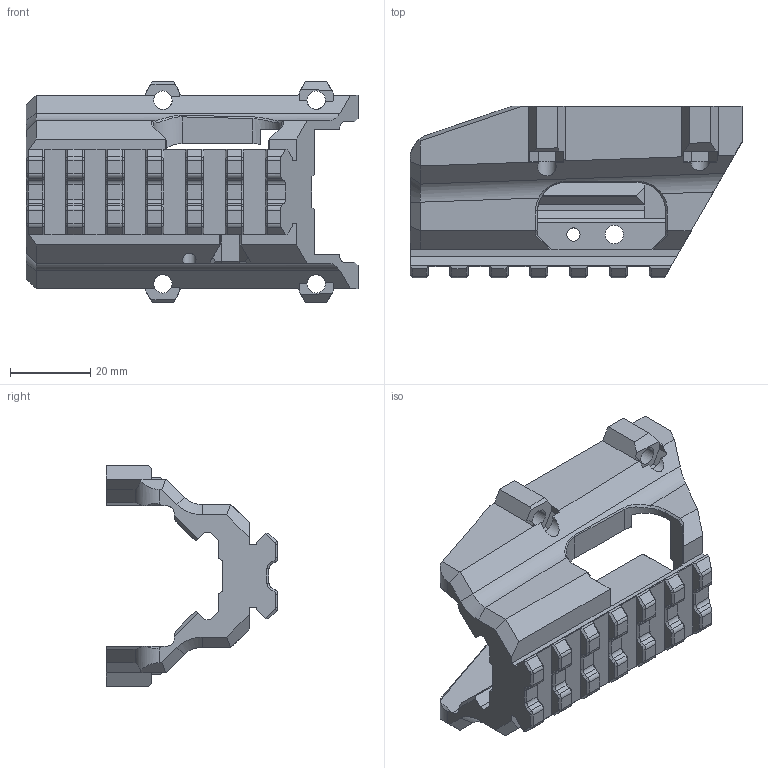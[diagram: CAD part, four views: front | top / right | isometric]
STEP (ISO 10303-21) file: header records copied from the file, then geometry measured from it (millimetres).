
FILE_DESCRIPTION (( 'STEP AP214' ), '1' );
FILE_NAME ('Chassis - Mount.STEP', '2022-02-04T02:39:33', ( '' ), ( '' ), 'SwSTEP 2.0', 'SolidWorks 2020', '' );
FILE_SCHEMA (( 'AUTOMOTIVE_DESIGN' ));
Length unit declared in the file: inch
Products named in the file (1): Chassis - Mount
Bounding box: 82.55 x 42.67 x 54.8 mm (x, y, z)
Volume: 42816.1 mm3; surface area: 19052.2 mm2
Topology: 1 solids, 1 shells, 488 faces, 1291 edges, 802 vertices
Faces by surface type: plane 320, cone 91, cylinder 72, bspline 5
Entity records: 15427 total; most frequent: CARTESIAN_POINT 3362, ORIENTED_EDGE 2582, DIRECTION 2414, EDGE_CURVE 1291, VECTOR 1004, LINE 1004, VERTEX_POINT 802, AXIS2_PLACEMENT_3D 705
